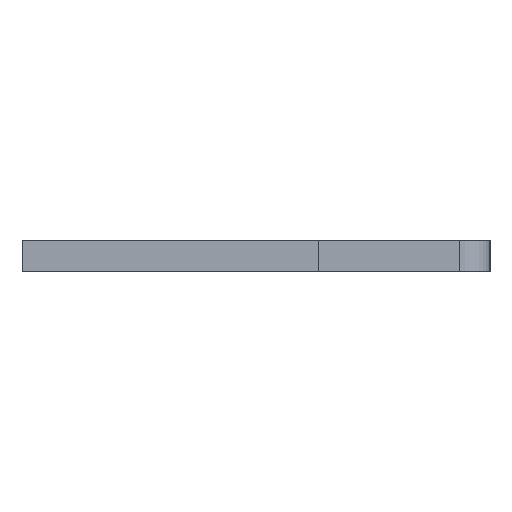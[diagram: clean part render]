
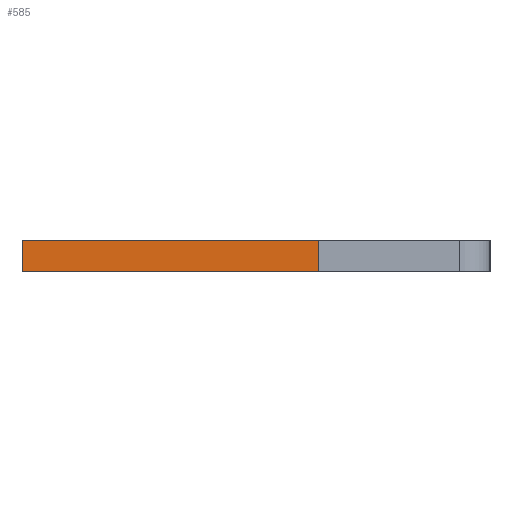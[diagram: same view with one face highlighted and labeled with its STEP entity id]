
A CAD part, left-side view. The second image highlights one B-rep face of the part: STEP entity #585.
In plain terms, the highlighted face is planar.
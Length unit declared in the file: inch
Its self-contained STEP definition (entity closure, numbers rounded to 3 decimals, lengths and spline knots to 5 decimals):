
#26 = DIRECTION ( 'NONE',  ( -1., 0., 0. ) ) ;
#47 = VERTEX_POINT ( 'NONE', #478 ) ;
#310 = ORIENTED_EDGE ( 'NONE', *, *, #546, .F. ) ;
#385 = DIRECTION ( 'NONE',  ( -1., 0., 0. ) ) ;
#475 = VERTEX_POINT ( 'NONE', #1437 ) ;
#478 = CARTESIAN_POINT ( 'NONE',  ( -0.01, 0.15, -0.04 ) ) ;
#514 = LINE ( 'NONE', #1298, #2032 ) ;
#525 = CARTESIAN_POINT ( 'NONE',  ( 0.01, 0.15, -0.04 ) ) ;
#532 = CARTESIAN_POINT ( 'NONE',  ( 0.01, 0.15, -0.04 ) ) ;
#546 = EDGE_CURVE ( 'NONE', #2226, #47, #1130, .T. ) ;
#569 = DIRECTION ( 'NONE',  ( 1., 0., 0. ) ) ;
#585 = ADVANCED_FACE ( 'NONE', ( #691 ), #1649, .F. ) ;
#691 = FACE_OUTER_BOUND ( 'NONE', #1692, .T. ) ;
#750 = EDGE_CURVE ( 'NONE', #1161, #475, #2059, .T. ) ;
#851 = ORIENTED_EDGE ( 'NONE', *, *, #1741, .F. ) ;
#860 = VECTOR ( 'NONE', #2142, 39.37008 ) ;
#863 = VECTOR ( 'NONE', #26, 39.37008 ) ;
#871 = EDGE_CURVE ( 'NONE', #475, #47, #514, .T. ) ;
#1043 = VECTOR ( 'NONE', #385, 39.37008 ) ;
#1130 = LINE ( 'NONE', #525, #1043 ) ;
#1161 = VERTEX_POINT ( 'NONE', #1750 ) ;
#1298 = CARTESIAN_POINT ( 'NONE',  ( -0.01, 0.15, -0.04 ) ) ;
#1312 = DIRECTION ( 'NONE',  ( 0., 1., 0. ) ) ;
#1437 = CARTESIAN_POINT ( 'NONE',  ( -0.01, -0.04, -0.04 ) ) ;
#1461 = ORIENTED_EDGE ( 'NONE', *, *, #750, .T. ) ;
#1490 = DIRECTION ( 'NONE',  ( 0., 0., 1. ) ) ;
#1649 = PLANE ( 'NONE',  #2081 ) ;
#1670 = CARTESIAN_POINT ( 'NONE',  ( 0.01, 0.15, -0.04 ) ) ;
#1671 = CARTESIAN_POINT ( 'NONE',  ( 0.01, 0.15, -0.04 ) ) ;
#1692 = EDGE_LOOP ( 'NONE', ( #1833, #310, #851, #1461 ) ) ;
#1730 = LINE ( 'NONE', #1671, #860 ) ;
#1741 = EDGE_CURVE ( 'NONE', #1161, #2226, #1730, .T. ) ;
#1750 = CARTESIAN_POINT ( 'NONE',  ( 0.01, -0.04, -0.04 ) ) ;
#1833 = ORIENTED_EDGE ( 'NONE', *, *, #871, .T. ) ;
#2029 = CARTESIAN_POINT ( 'NONE',  ( 0.01, -0.04, -0.04 ) ) ;
#2032 = VECTOR ( 'NONE', #1312, 39.37008 ) ;
#2059 = LINE ( 'NONE', #2029, #863 ) ;
#2081 = AXIS2_PLACEMENT_3D ( 'NONE', #1670, #1490, #569 ) ;
#2142 = DIRECTION ( 'NONE',  ( 0., 1., 0. ) ) ;
#2226 = VERTEX_POINT ( 'NONE', #532 ) ;
